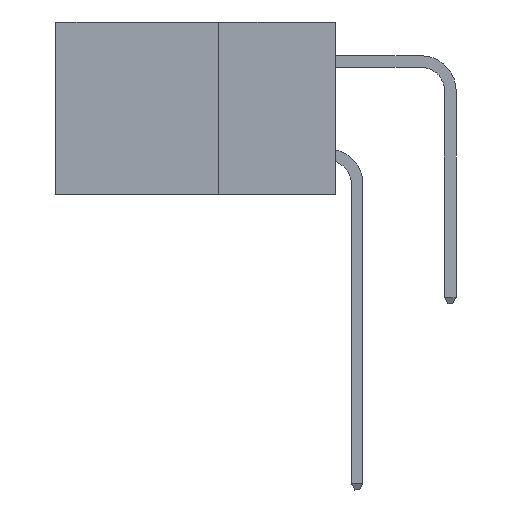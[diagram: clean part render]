
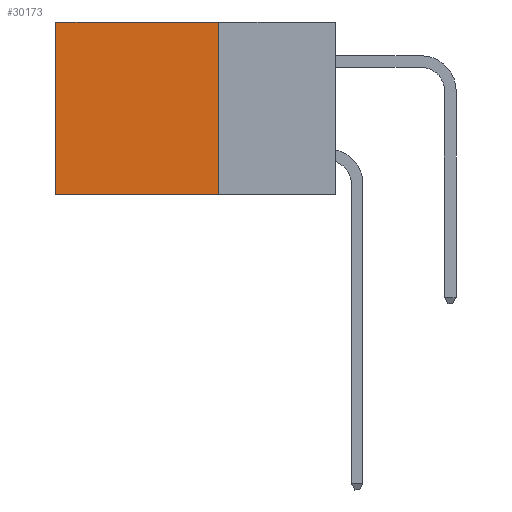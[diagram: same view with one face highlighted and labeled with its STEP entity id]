
A CAD part, left-side view. The second image highlights one B-rep face of the part: STEP entity #30173.
In plain terms, the highlighted planar face has unit normal (-1, 0, 0).
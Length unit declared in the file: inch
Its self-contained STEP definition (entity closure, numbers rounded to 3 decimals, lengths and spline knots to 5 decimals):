
#641 = VERTEX_POINT ( 'NONE', #17326 ) ;
#1670 = DIRECTION ( 'NONE',  ( 0., 0., -1. ) ) ;
#2680 = EDGE_CURVE ( 'NONE', #641, #34103, #20403, .T. ) ;
#9835 = DIRECTION ( 'NONE',  ( 0., 0., -1. ) ) ;
#12945 = ORIENTED_EDGE ( 'NONE', *, *, #28770, .T. ) ;
#12946 = FACE_OUTER_BOUND ( 'NONE', #22427, .T. ) ;
#13752 = ORIENTED_EDGE ( 'NONE', *, *, #25821, .F. ) ;
#14049 = DIRECTION ( 'NONE',  ( 0., 0., -1. ) ) ;
#15070 = LINE ( 'NONE', #37727, #23356 ) ;
#15784 = ORIENTED_EDGE ( 'NONE', *, *, #2680, .T. ) ;
#15888 = AXIS2_PLACEMENT_3D ( 'NONE', #29868, #35922, #9835 ) ;
#17326 = CARTESIAN_POINT ( 'NONE',  ( 0.2875, 0.6, 0. ) ) ;
#17779 = CARTESIAN_POINT ( 'NONE',  ( 0.2875, 0.6, 0. ) ) ;
#19159 = VECTOR ( 'NONE', #14049, 39.37008 ) ;
#19777 = VECTOR ( 'NONE', #24918, 39.37008 ) ;
#20403 = LINE ( 'NONE', #17779, #32860 ) ;
#20933 = DIRECTION ( 'NONE',  ( 0., 1., 0. ) ) ;
#21340 = CARTESIAN_POINT ( 'NONE',  ( 0.2875, 0.25, -0.37 ) ) ;
#22427 = EDGE_LOOP ( 'NONE', ( #15784, #13752, #28046, #12945 ) ) ;
#23356 = VECTOR ( 'NONE', #20933, 39.37008 ) ;
#24918 = DIRECTION ( 'NONE',  ( 0., 1., 0. ) ) ;
#25449 = VERTEX_POINT ( 'NONE', #33712 ) ;
#25821 = EDGE_CURVE ( 'NONE', #40472, #34103, #15070, .T. ) ;
#26471 = EDGE_CURVE ( 'NONE', #25449, #40472, #34198, .T. ) ;
#28046 = ORIENTED_EDGE ( 'NONE', *, *, #26471, .F. ) ;
#28770 = EDGE_CURVE ( 'NONE', #25449, #641, #32229, .T. ) ;
#29868 = CARTESIAN_POINT ( 'NONE',  ( 0.2875, 0.25, 0. ) ) ;
#30173 = ADVANCED_FACE ( 'NONE', ( #12946 ), #42794, .F. ) ;
#32160 = CARTESIAN_POINT ( 'NONE',  ( 0.2875, 0.25, 0. ) ) ;
#32229 = LINE ( 'NONE', #32160, #19777 ) ;
#32860 = VECTOR ( 'NONE', #1670, 39.37008 ) ;
#33712 = CARTESIAN_POINT ( 'NONE',  ( 0.2875, 0.25, 0. ) ) ;
#33907 = CARTESIAN_POINT ( 'NONE',  ( 0.2875, 0.25, 0. ) ) ;
#34103 = VERTEX_POINT ( 'NONE', #39596 ) ;
#34198 = LINE ( 'NONE', #33907, #19159 ) ;
#35922 = DIRECTION ( 'NONE',  ( 1., 0., 0. ) ) ;
#37727 = CARTESIAN_POINT ( 'NONE',  ( 0.2875, 0.25, -0.37 ) ) ;
#39596 = CARTESIAN_POINT ( 'NONE',  ( 0.2875, 0.6, -0.37 ) ) ;
#40472 = VERTEX_POINT ( 'NONE', #21340 ) ;
#42794 = PLANE ( 'NONE',  #15888 ) ;
